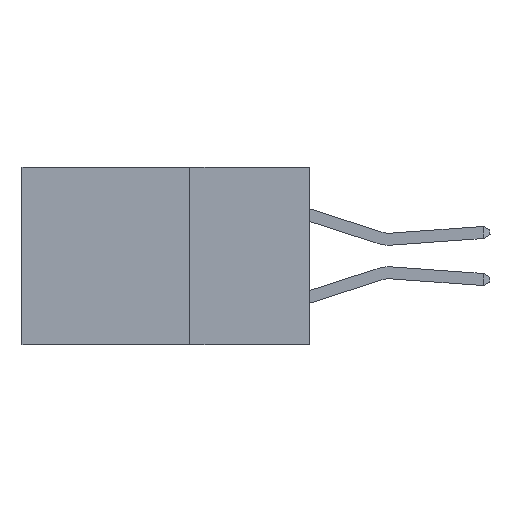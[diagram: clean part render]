
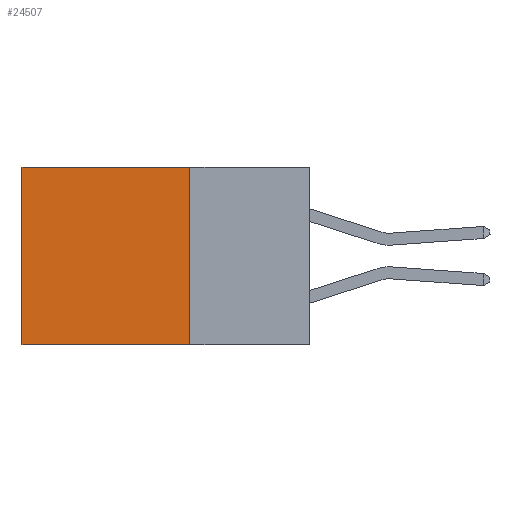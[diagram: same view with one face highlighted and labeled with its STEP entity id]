
A CAD part, left-side view. The second image highlights one B-rep face of the part: STEP entity #24507.
In plain terms, the highlighted planar face has unit normal (-1, 0, 0).
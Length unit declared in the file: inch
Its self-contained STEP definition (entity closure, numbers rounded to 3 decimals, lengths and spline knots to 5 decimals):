
#834 = CARTESIAN_POINT ( 'NONE',  ( 0.2615, 0.6, -0.37 ) ) ;
#963 = DIRECTION ( 'NONE',  ( 0., 0., -1. ) ) ;
#1681 = CARTESIAN_POINT ( 'NONE',  ( 0.2615, 0.25, 0. ) ) ;
#2913 = LINE ( 'NONE', #8992, #15851 ) ;
#3369 = CARTESIAN_POINT ( 'NONE',  ( 0.2615, 0.25, -0.37 ) ) ;
#3467 = VECTOR ( 'NONE', #963, 39.37008 ) ;
#4027 = CARTESIAN_POINT ( 'NONE',  ( 0.2615, 0.6, -0.37 ) ) ;
#4319 = EDGE_LOOP ( 'NONE', ( #9904, #24955, #8416, #8361 ) ) ;
#4661 = CARTESIAN_POINT ( 'NONE',  ( 0.2615, 0.6, 0. ) ) ;
#5073 = DIRECTION ( 'NONE',  ( 0., 0., -1. ) ) ;
#7035 = CARTESIAN_POINT ( 'NONE',  ( 0.2615, 0.25, -0.37 ) ) ;
#7231 = LINE ( 'NONE', #15165, #24031 ) ;
#8361 = ORIENTED_EDGE ( 'NONE', *, *, #21987, .T. ) ;
#8416 = ORIENTED_EDGE ( 'NONE', *, *, #21929, .F. ) ;
#8992 = CARTESIAN_POINT ( 'NONE',  ( 0.2615, 0.25, -0.37 ) ) ;
#9081 = AXIS2_PLACEMENT_3D ( 'NONE', #7035, #13211, #15225 ) ;
#9696 = LINE ( 'NONE', #17888, #18063 ) ;
#9904 = ORIENTED_EDGE ( 'NONE', *, *, #24105, .T. ) ;
#10270 = VERTEX_POINT ( 'NONE', #4027 ) ;
#10518 = VERTEX_POINT ( 'NONE', #4661 ) ;
#11350 = LINE ( 'NONE', #834, #3467 ) ;
#13211 = DIRECTION ( 'NONE',  ( 1., 0., 0. ) ) ;
#13410 = DIRECTION ( 'NONE',  ( 0., 1., 0. ) ) ;
#15165 = CARTESIAN_POINT ( 'NONE',  ( 0.2615, 0.25, 0. ) ) ;
#15225 = DIRECTION ( 'NONE',  ( 0., 0., -1. ) ) ;
#15851 = VECTOR ( 'NONE', #5073, 39.37008 ) ;
#17121 = PLANE ( 'NONE',  #9081 ) ;
#17661 = EDGE_CURVE ( 'NONE', #20950, #10270, #9696, .T. ) ;
#17888 = CARTESIAN_POINT ( 'NONE',  ( 0.2615, 0.25, -0.37 ) ) ;
#18063 = VECTOR ( 'NONE', #26134, 39.37008 ) ;
#20950 = VERTEX_POINT ( 'NONE', #3369 ) ;
#21929 = EDGE_CURVE ( 'NONE', #22140, #20950, #2913, .T. ) ;
#21987 = EDGE_CURVE ( 'NONE', #22140, #10518, #7231, .T. ) ;
#22140 = VERTEX_POINT ( 'NONE', #1681 ) ;
#24031 = VECTOR ( 'NONE', #13410, 39.37008 ) ;
#24105 = EDGE_CURVE ( 'NONE', #10518, #10270, #11350, .T. ) ;
#24507 = ADVANCED_FACE ( 'NONE', ( #24826 ), #17121, .F. ) ;
#24826 = FACE_OUTER_BOUND ( 'NONE', #4319, .T. ) ;
#24955 = ORIENTED_EDGE ( 'NONE', *, *, #17661, .F. ) ;
#26134 = DIRECTION ( 'NONE',  ( 0., 1., 0. ) ) ;
